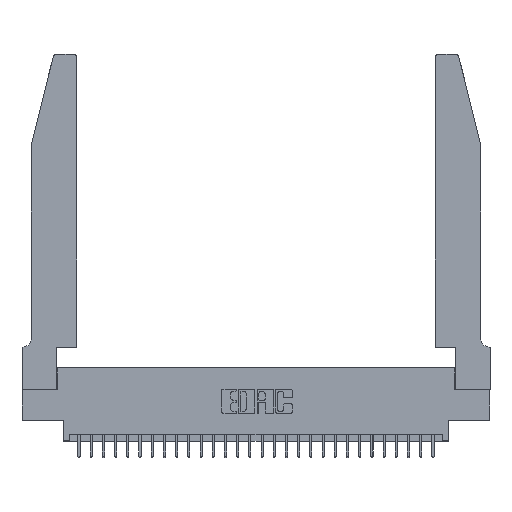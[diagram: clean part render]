
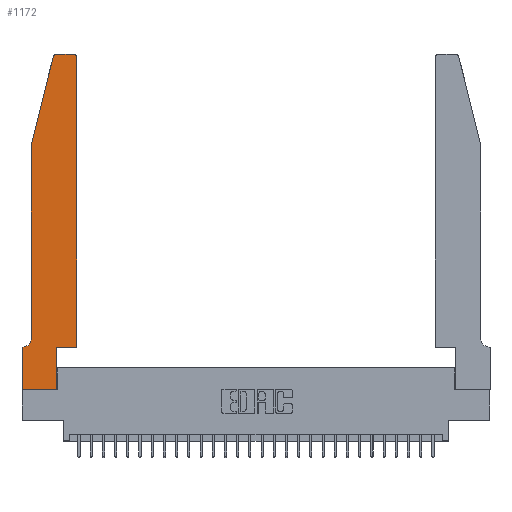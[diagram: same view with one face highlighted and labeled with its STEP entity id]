
A CAD part, top view. The second image highlights one B-rep face of the part: STEP entity #1172.
In plain terms, the highlighted planar face has unit normal (0, 0, 1).
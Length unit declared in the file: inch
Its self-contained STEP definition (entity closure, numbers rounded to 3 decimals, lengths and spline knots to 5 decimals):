
#871 = CARTESIAN_POINT ( 'NONE',  ( 0.4505, 0.35, 0.37 ) ) ;
#927 = EDGE_CURVE ( 'NONE', #3807, #24017, #26785, .T. ) ;
#1013 = DIRECTION ( 'NONE',  ( -0.239, -0.971, 0. ) ) ;
#1072 = EDGE_CURVE ( 'NONE', #18229, #20250, #14947, .T. ) ;
#1153 = DIRECTION ( 'NONE',  ( 1., 0., 0. ) ) ;
#1163 = LINE ( 'NONE', #26323, #15026 ) ;
#1172 = ADVANCED_FACE ( 'NONE', ( #20288 ), #26895, .T. ) ;
#1365 = ORIENTED_EDGE ( 'NONE', *, *, #25623, .T. ) ;
#1420 = DIRECTION ( 'NONE',  ( 0., 1., 0. ) ) ;
#1643 = DIRECTION ( 'NONE',  ( -1., 0., 0. ) ) ;
#2870 = VECTOR ( 'NONE', #27484, 39.37008 ) ;
#3807 = VERTEX_POINT ( 'NONE', #13398 ) ;
#4290 = EDGE_CURVE ( 'NONE', #15103, #18229, #18624, .T. ) ;
#4723 = DIRECTION ( 'NONE',  ( 0., -1., 0. ) ) ;
#5094 = CARTESIAN_POINT ( 'NONE',  ( 0.0755, 0.35, 0.37 ) ) ;
#5169 = DIRECTION ( 'NONE',  ( 0., 1., 0. ) ) ;
#5567 = CARTESIAN_POINT ( 'NONE',  ( 0.4205, 2.72, 0.37 ) ) ;
#5593 = VECTOR ( 'NONE', #7561, 39.37008 ) ;
#5609 = CIRCLE ( 'NONE', #6109, 0.03 ) ;
#6000 = DIRECTION ( 'NONE',  ( 1., 0., 0. ) ) ;
#6109 = AXIS2_PLACEMENT_3D ( 'NONE', #5567, #8284, #1153 ) ;
#6210 = LINE ( 'NONE', #15745, #28107 ) ;
#6703 = VERTEX_POINT ( 'NONE', #12790 ) ;
#6724 = CARTESIAN_POINT ( 'NONE',  ( 0.4505, 0.35, 0.37 ) ) ;
#6798 = VERTEX_POINT ( 'NONE', #9922 ) ;
#7561 = DIRECTION ( 'NONE',  ( 1., 0., 0. ) ) ;
#7687 = CARTESIAN_POINT ( 'NONE',  ( 0., 0., 0.37 ) ) ;
#7991 = CARTESIAN_POINT ( 'NONE',  ( 0.4505, 0.35, 0.37 ) ) ;
#8284 = DIRECTION ( 'NONE',  ( 0., 0., 1. ) ) ;
#8463 = VERTEX_POINT ( 'NONE', #28115 ) ;
#8514 = LINE ( 'NONE', #26720, #9672 ) ;
#9050 = ORIENTED_EDGE ( 'NONE', *, *, #1072, .T. ) ;
#9266 = LINE ( 'NONE', #18561, #19613 ) ;
#9503 = VERTEX_POINT ( 'NONE', #19035 ) ;
#9641 = ORIENTED_EDGE ( 'NONE', *, *, #20480, .T. ) ;
#9672 = VECTOR ( 'NONE', #1420, 39.37008 ) ;
#9922 = CARTESIAN_POINT ( 'NONE',  ( 0.2865, 0., 0.37 ) ) ;
#10975 = DIRECTION ( 'NONE',  ( 0., 0., 1. ) ) ;
#11561 = EDGE_CURVE ( 'NONE', #8463, #9503, #9266, .T. ) ;
#11815 = ORIENTED_EDGE ( 'NONE', *, *, #21131, .T. ) ;
#12065 = DIRECTION ( 'NONE',  ( 0., -1., 0. ) ) ;
#12790 = CARTESIAN_POINT ( 'NONE',  ( 0.4205, 2.75, 0.37 ) ) ;
#13298 = CARTESIAN_POINT ( 'NONE',  ( 0.0055, 0.35, 0.37 ) ) ;
#13398 = CARTESIAN_POINT ( 'NONE',  ( 0.284, 2.75, 0.37 ) ) ;
#14040 = DIRECTION ( 'NONE',  ( 1., 0., 0. ) ) ;
#14837 = LINE ( 'NONE', #871, #5593 ) ;
#14947 = LINE ( 'NONE', #7687, #29687 ) ;
#14960 = VECTOR ( 'NONE', #5169, 39.37008 ) ;
#15026 = VECTOR ( 'NONE', #1013, 39.37008 ) ;
#15103 = VERTEX_POINT ( 'NONE', #13298 ) ;
#15330 = CARTESIAN_POINT ( 'NONE',  ( 0.25487, 2.72718, 0.37 ) ) ;
#15368 = CARTESIAN_POINT ( 'NONE',  ( 0.4505, 2.72, 0.37 ) ) ;
#15399 = ORIENTED_EDGE ( 'NONE', *, *, #11561, .T. ) ;
#15496 = AXIS2_PLACEMENT_3D ( 'NONE', #17993, #10975, #6000 ) ;
#15717 = VERTEX_POINT ( 'NONE', #15368 ) ;
#15745 = CARTESIAN_POINT ( 'NONE',  ( 0.2605, 2.75, 0.37 ) ) ;
#16189 = CARTESIAN_POINT ( 'NONE',  ( 0., 0.35, 0.37 ) ) ;
#16326 = DIRECTION ( 'NONE',  ( -1., 0., 0. ) ) ;
#16531 = ORIENTED_EDGE ( 'NONE', *, *, #927, .T. ) ;
#16550 = CARTESIAN_POINT ( 'NONE',  ( 0., 0., 0.37 ) ) ;
#16976 = AXIS2_PLACEMENT_3D ( 'NONE', #30127, #27838, #14040 ) ;
#17451 = EDGE_CURVE ( 'NONE', #6703, #3807, #6210, .T. ) ;
#17750 = ORIENTED_EDGE ( 'NONE', *, *, #4290, .T. ) ;
#17897 = CARTESIAN_POINT ( 'NONE',  ( 0., 0., 0.37 ) ) ;
#17993 = CARTESIAN_POINT ( 'NONE',  ( 0., 0.35, 0.37 ) ) ;
#18229 = VERTEX_POINT ( 'NONE', #16189 ) ;
#18530 = VERTEX_POINT ( 'NONE', #7991 ) ;
#18561 = CARTESIAN_POINT ( 'NONE',  ( 0.0755, 2., 0.37 ) ) ;
#18624 = LINE ( 'NONE', #5094, #23826 ) ;
#18629 = CARTESIAN_POINT ( 'NONE',  ( 0.0055, 0.42, 0.37 ) ) ;
#18842 = LINE ( 'NONE', #16550, #2870 ) ;
#19035 = CARTESIAN_POINT ( 'NONE',  ( 0.0755, 0.42, 0.37 ) ) ;
#19324 = ORIENTED_EDGE ( 'NONE', *, *, #24626, .T. ) ;
#19573 = EDGE_CURVE ( 'NONE', #9503, #15103, #29636, .T. ) ;
#19613 = VECTOR ( 'NONE', #4723, 39.37008 ) ;
#20097 = EDGE_LOOP ( 'NONE', ( #20338, #16531, #9641, #15399, #29149, #17750, #9050, #27090, #22619, #19324, #11815, #1365 ) ) ;
#20250 = VERTEX_POINT ( 'NONE', #17897 ) ;
#20288 = FACE_OUTER_BOUND ( 'NONE', #20097, .T. ) ;
#20338 = ORIENTED_EDGE ( 'NONE', *, *, #17451, .T. ) ;
#20480 = EDGE_CURVE ( 'NONE', #24017, #8463, #1163, .T. ) ;
#21131 = EDGE_CURVE ( 'NONE', #18530, #15717, #23479, .T. ) ;
#21245 = EDGE_CURVE ( 'NONE', #20250, #6798, #18842, .T. ) ;
#22048 = VERTEX_POINT ( 'NONE', #26444 ) ;
#22304 = AXIS2_PLACEMENT_3D ( 'NONE', #18629, #26146, #16326 ) ;
#22619 = ORIENTED_EDGE ( 'NONE', *, *, #29685, .T. ) ;
#23479 = LINE ( 'NONE', #6724, #14960 ) ;
#23826 = VECTOR ( 'NONE', #25834, 39.37008 ) ;
#24017 = VERTEX_POINT ( 'NONE', #15330 ) ;
#24626 = EDGE_CURVE ( 'NONE', #22048, #18530, #14837, .T. ) ;
#25623 = EDGE_CURVE ( 'NONE', #15717, #6703, #5609, .T. ) ;
#25834 = DIRECTION ( 'NONE',  ( -1., 0., 0. ) ) ;
#26146 = DIRECTION ( 'NONE',  ( 0., 0., -1. ) ) ;
#26323 = CARTESIAN_POINT ( 'NONE',  ( 0.0755, 2., 0.37 ) ) ;
#26444 = CARTESIAN_POINT ( 'NONE',  ( 0.2865, 0.35, 0.37 ) ) ;
#26720 = CARTESIAN_POINT ( 'NONE',  ( 0.2865, 0.35, 0.37 ) ) ;
#26785 = CIRCLE ( 'NONE', #16976, 0.03 ) ;
#26895 = PLANE ( 'NONE',  #15496 ) ;
#27090 = ORIENTED_EDGE ( 'NONE', *, *, #21245, .T. ) ;
#27484 = DIRECTION ( 'NONE',  ( 1., 0., 0. ) ) ;
#27838 = DIRECTION ( 'NONE',  ( 0., 0., 1. ) ) ;
#28107 = VECTOR ( 'NONE', #1643, 39.37008 ) ;
#28115 = CARTESIAN_POINT ( 'NONE',  ( 0.0755, 2., 0.37 ) ) ;
#29149 = ORIENTED_EDGE ( 'NONE', *, *, #19573, .T. ) ;
#29636 = CIRCLE ( 'NONE', #22304, 0.07 ) ;
#29685 = EDGE_CURVE ( 'NONE', #6798, #22048, #8514, .T. ) ;
#29687 = VECTOR ( 'NONE', #12065, 39.37008 ) ;
#30127 = CARTESIAN_POINT ( 'NONE',  ( 0.284, 2.72, 0.37 ) ) ;
